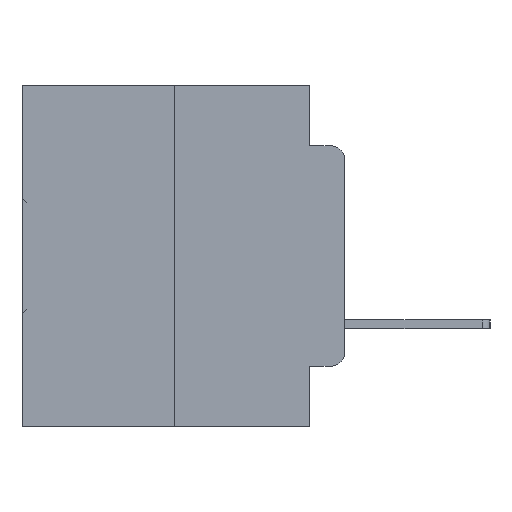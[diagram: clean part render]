
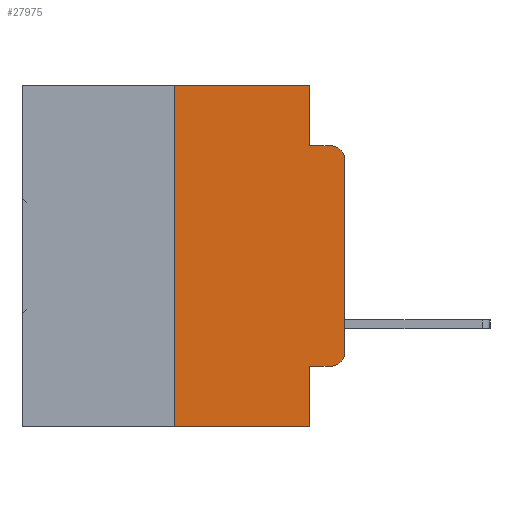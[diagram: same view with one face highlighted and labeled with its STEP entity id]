
A CAD part, left-side view. The second image highlights one B-rep face of the part: STEP entity #27975.
In plain terms, the highlighted planar face has unit normal (-1, 0, 0).
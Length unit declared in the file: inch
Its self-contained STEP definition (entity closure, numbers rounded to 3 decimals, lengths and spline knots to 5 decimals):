
#29 = VECTOR ( 'NONE', #29486, 39.37008 ) ;
#97 = CARTESIAN_POINT ( 'NONE',  ( 0., 0.02, -0.4115 ) ) ;
#439 = CARTESIAN_POINT ( 'NONE',  ( 0., 0.051, 0. ) ) ;
#1032 = CARTESIAN_POINT ( 'NONE',  ( 0., 0.473, -0.5 ) ) ;
#1605 = DIRECTION ( 'NONE',  ( -1., 0., 0. ) ) ;
#2209 = VERTEX_POINT ( 'NONE', #31357 ) ;
#2830 = LINE ( 'NONE', #7790, #9080 ) ;
#3365 = CARTESIAN_POINT ( 'NONE',  ( 0., 0.02, -0.0885 ) ) ;
#4182 = CARTESIAN_POINT ( 'NONE',  ( 0., 0.051, 0. ) ) ;
#4282 = EDGE_CURVE ( 'NONE', #25612, #19971, #2830, .T. ) ;
#4706 = ORIENTED_EDGE ( 'NONE', *, *, #29363, .T. ) ;
#4865 = AXIS2_PLACEMENT_3D ( 'NONE', #10328, #33767, #18417 ) ;
#4952 = PLANE ( 'NONE',  #4865 ) ;
#5244 = DIRECTION ( 'NONE',  ( 0., -1., 0. ) ) ;
#5487 = LINE ( 'NONE', #1032, #11774 ) ;
#5547 = DIRECTION ( 'NONE',  ( 0., 0., 1. ) ) ;
#5985 = CARTESIAN_POINT ( 'NONE',  ( 0., 0.02, -0.3915 ) ) ;
#6147 = VERTEX_POINT ( 'NONE', #30463 ) ;
#6225 = CARTESIAN_POINT ( 'NONE',  ( 0., 0.051, 0. ) ) ;
#7201 = ORIENTED_EDGE ( 'NONE', *, *, #4282, .F. ) ;
#7627 = ORIENTED_EDGE ( 'NONE', *, *, #24129, .F. ) ;
#7790 = CARTESIAN_POINT ( 'NONE',  ( 0., 0.051, -0.0885 ) ) ;
#8062 = ORIENTED_EDGE ( 'NONE', *, *, #9537, .T. ) ;
#8156 = LINE ( 'NONE', #26504, #27633 ) ;
#8671 = DIRECTION ( 'NONE',  ( 0., 0., -1. ) ) ;
#9080 = VECTOR ( 'NONE', #13237, 39.37008 ) ;
#9500 = DIRECTION ( 'NONE',  ( 0., 0., 1. ) ) ;
#9537 = EDGE_CURVE ( 'NONE', #30178, #13573, #8156, .T. ) ;
#9547 = VECTOR ( 'NONE', #24647, 39.37008 ) ;
#9917 = EDGE_CURVE ( 'NONE', #33279, #19971, #30754, .T. ) ;
#10328 = CARTESIAN_POINT ( 'NONE',  ( 0., 0.473, 0. ) ) ;
#11774 = VECTOR ( 'NONE', #27477, 39.37008 ) ;
#12271 = FACE_OUTER_BOUND ( 'NONE', #14054, .T. ) ;
#13237 = DIRECTION ( 'NONE',  ( 0., -1., 0. ) ) ;
#13244 = EDGE_CURVE ( 'NONE', #23712, #6147, #5487, .T. ) ;
#13573 = VERTEX_POINT ( 'NONE', #97 ) ;
#13648 = EDGE_CURVE ( 'NONE', #21546, #25612, #28248, .T. ) ;
#14054 = EDGE_LOOP ( 'NONE', ( #4706, #27517, #7201, #24697, #7627, #28745, #18144, #19788, #8062, #33023 ) ) ;
#14282 = EDGE_CURVE ( 'NONE', #30178, #6147, #32849, .T. ) ;
#14896 = CARTESIAN_POINT ( 'NONE',  ( 0., 0.25, -0.5 ) ) ;
#15397 = EDGE_CURVE ( 'NONE', #13573, #32538, #34016, .T. ) ;
#16718 = CARTESIAN_POINT ( 'NONE',  ( 0., 0.473, 0. ) ) ;
#16780 = CARTESIAN_POINT ( 'NONE',  ( 0., 0., -0.3915 ) ) ;
#17650 = CARTESIAN_POINT ( 'NONE',  ( 0., 0.02, -0.1085 ) ) ;
#18144 = ORIENTED_EDGE ( 'NONE', *, *, #13244, .T. ) ;
#18417 = DIRECTION ( 'NONE',  ( 0., 0., -1. ) ) ;
#19229 = VECTOR ( 'NONE', #19795, 39.37008 ) ;
#19788 = ORIENTED_EDGE ( 'NONE', *, *, #14282, .F. ) ;
#19795 = DIRECTION ( 'NONE',  ( 0., 0., -1. ) ) ;
#19971 = VERTEX_POINT ( 'NONE', #3365 ) ;
#20296 = DIRECTION ( 'NONE',  ( 0., 0., -1. ) ) ;
#20757 = AXIS2_PLACEMENT_3D ( 'NONE', #17650, #1605, #20296 ) ;
#21546 = VERTEX_POINT ( 'NONE', #4182 ) ;
#23217 = CARTESIAN_POINT ( 'NONE',  ( 0., 0.051, -0.4115 ) ) ;
#23712 = VERTEX_POINT ( 'NONE', #14896 ) ;
#24070 = CARTESIAN_POINT ( 'NONE',  ( 0., 0., 0. ) ) ;
#24129 = EDGE_CURVE ( 'NONE', #2209, #21546, #31279, .T. ) ;
#24609 = DIRECTION ( 'NONE',  ( -1., 0., 0. ) ) ;
#24647 = DIRECTION ( 'NONE',  ( 0., -1., 0. ) ) ;
#24697 = ORIENTED_EDGE ( 'NONE', *, *, #13648, .F. ) ;
#24901 = EDGE_CURVE ( 'NONE', #23712, #2209, #31969, .T. ) ;
#25421 = LINE ( 'NONE', #24070, #29812 ) ;
#25612 = VERTEX_POINT ( 'NONE', #26071 ) ;
#26071 = CARTESIAN_POINT ( 'NONE',  ( 0., 0.051, -0.0885 ) ) ;
#26104 = VECTOR ( 'NONE', #9500, 39.37008 ) ;
#26504 = CARTESIAN_POINT ( 'NONE',  ( 0., 0.051, -0.4115 ) ) ;
#26748 = CARTESIAN_POINT ( 'NONE',  ( 0., 0., -0.1085 ) ) ;
#27477 = DIRECTION ( 'NONE',  ( 0., -1., 0. ) ) ;
#27517 = ORIENTED_EDGE ( 'NONE', *, *, #9917, .T. ) ;
#27633 = VECTOR ( 'NONE', #5244, 39.37008 ) ;
#27975 = ADVANCED_FACE ( 'NONE', ( #12271 ), #4952, .F. ) ;
#27996 = CARTESIAN_POINT ( 'NONE',  ( 0., 0.25, 0. ) ) ;
#28248 = LINE ( 'NONE', #439, #29 ) ;
#28745 = ORIENTED_EDGE ( 'NONE', *, *, #24901, .F. ) ;
#29363 = EDGE_CURVE ( 'NONE', #32538, #33279, #25421, .T. ) ;
#29486 = DIRECTION ( 'NONE',  ( 0., 0., -1. ) ) ;
#29812 = VECTOR ( 'NONE', #5547, 39.37008 ) ;
#30178 = VERTEX_POINT ( 'NONE', #23217 ) ;
#30463 = CARTESIAN_POINT ( 'NONE',  ( 0., 0.051, -0.5 ) ) ;
#30754 = CIRCLE ( 'NONE', #20757, 0.02 ) ;
#31279 = LINE ( 'NONE', #16718, #9547 ) ;
#31357 = CARTESIAN_POINT ( 'NONE',  ( 0., 0.25, 0. ) ) ;
#31594 = AXIS2_PLACEMENT_3D ( 'NONE', #5985, #24609, #8671 ) ;
#31969 = LINE ( 'NONE', #27996, #26104 ) ;
#32538 = VERTEX_POINT ( 'NONE', #16780 ) ;
#32849 = LINE ( 'NONE', #6225, #19229 ) ;
#33023 = ORIENTED_EDGE ( 'NONE', *, *, #15397, .T. ) ;
#33279 = VERTEX_POINT ( 'NONE', #26748 ) ;
#33767 = DIRECTION ( 'NONE',  ( 1., 0., 0. ) ) ;
#34016 = CIRCLE ( 'NONE', #31594, 0.02 ) ;
